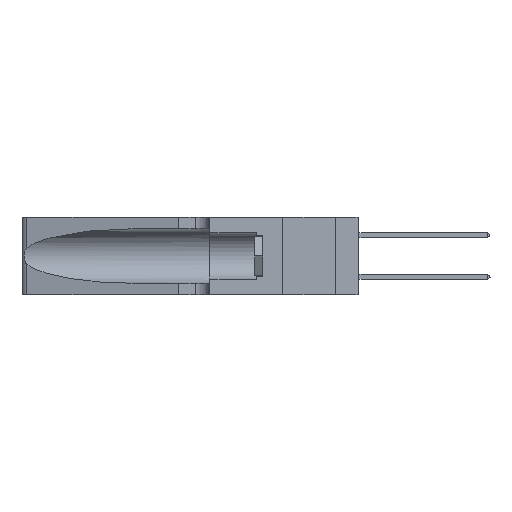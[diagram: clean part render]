
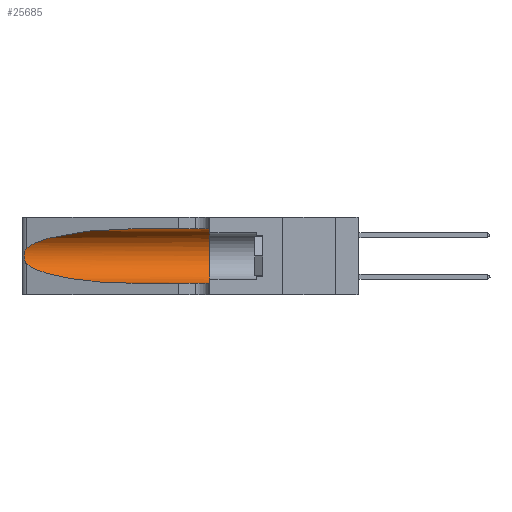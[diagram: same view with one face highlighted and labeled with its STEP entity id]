
A CAD part, left-side view. The second image highlights one B-rep face of the part: STEP entity #25685.
In plain terms, the highlighted cylindrical face has radius 3.308 mm (diameter 6.617 mm), a partial arc.
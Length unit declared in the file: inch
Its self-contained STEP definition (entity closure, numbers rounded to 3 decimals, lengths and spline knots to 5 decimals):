
#281 = CARTESIAN_POINT ( 'NONE',  ( 0.18966, 0.96281, 0.31525 ) ) ;
#1956 = CARTESIAN_POINT ( 'NONE',  ( 0.1305, 0.35, 0.185 ) ) ;
#2279 = VERTEX_POINT ( 'NONE', #17155 ) ;
#3001 = CARTESIAN_POINT ( 'NONE',  ( 0.25639, 1.23186, 0.15144 ) ) ;
#3052 = VERTEX_POINT ( 'NONE', #40512 ) ;
#3433 = VERTEX_POINT ( 'NONE', #13329 ) ;
#3722 = VERTEX_POINT ( 'NONE', #3764 ) ;
#3764 = CARTESIAN_POINT ( 'NONE',  ( 0.1305, 0.72297, 0.05475 ) ) ;
#4044 = ORIENTED_EDGE ( 'NONE', *, *, #33593, .T. ) ;
#4842 =( BOUNDED_CURVE ( )  B_SPLINE_CURVE ( 3, ( #26065, #281, #37174, #15163 ),
 .UNSPECIFIED., .F., .F. ) 
 B_SPLINE_CURVE_WITH_KNOTS ( ( 4, 4 ),
 ( 1.5708, 2.84003 ),
 .UNSPECIFIED. ) 
 CURVE ( )  GEOMETRIC_REPRESENTATION_ITEM ( )  RATIONAL_B_SPLINE_CURVE ( ( 1., 0.87, 0.87, 1. ) ) 
 REPRESENTATION_ITEM ( '' )  );
#5700 = DIRECTION ( 'NONE',  ( 0., 0., 1. ) ) ;
#6521 = CIRCLE ( 'NONE', #29920, 0.13025 ) ;
#6698 = AXIS2_PLACEMENT_3D ( 'NONE', #32342, #10132, #10285 ) ;
#6740 = CARTESIAN_POINT ( 'NONE',  ( 0.25487, 1.22718, 0.14631 ) ) ;
#8478 = VERTEX_POINT ( 'NONE', #41001 ) ;
#8802 = EDGE_CURVE ( 'NONE', #44204, #3433, #39065, .T. ) ;
#9090 = ORIENTED_EDGE ( 'NONE', *, *, #8802, .T. ) ;
#10132 = DIRECTION ( 'NONE',  ( 0., -1., 0. ) ) ;
#10261 = CARTESIAN_POINT ( 'NONE',  ( 0.25639, 1.23184, 0.21858 ) ) ;
#10285 = DIRECTION ( 'NONE',  ( 0., 0., -1. ) ) ;
#11110 = CARTESIAN_POINT ( 'NONE',  ( 0.18966, 0.96281, 0.05475 ) ) ;
#13057 = VECTOR ( 'NONE', #42154, 39.37008 ) ;
#13329 = CARTESIAN_POINT ( 'NONE',  ( 0.25487, 1.22718, 0.14631 ) ) ;
#13637 = VECTOR ( 'NONE', #43519, 39.37008 ) ;
#13995 = CARTESIAN_POINT ( 'NONE',  ( 0.25854, 1.2359, 0.20912 ) ) ;
#14206 = LINE ( 'NONE', #34748, #13057 ) ;
#15163 = CARTESIAN_POINT ( 'NONE',  ( 0.25487, 1.22718, 0.22369 ) ) ;
#17155 = CARTESIAN_POINT ( 'NONE',  ( 0.1305, 0.35, 0.05475 ) ) ;
#17729 = CARTESIAN_POINT ( 'NONE',  ( 0.26075, 1.23896, 0.19203 ) ) ;
#18454 =( BOUNDED_CURVE ( )  B_SPLINE_CURVE ( 3, ( #29433, #33156, #11110, #36834 ),
 .UNSPECIFIED., .F., .F. ) 
 B_SPLINE_CURVE_WITH_KNOTS ( ( 4, 4 ),
 ( 3.44316, 4.71239 ),
 .UNSPECIFIED. ) 
 CURVE ( )  GEOMETRIC_REPRESENTATION_ITEM ( )  RATIONAL_B_SPLINE_CURVE ( ( 1., 0.87, 0.87, 1. ) ) 
 REPRESENTATION_ITEM ( '' )  );
#19621 = EDGE_CURVE ( 'NONE', #3722, #2279, #23403, .T. ) ;
#21366 = CARTESIAN_POINT ( 'NONE',  ( 0.26017, 1.23833, 0.17102 ) ) ;
#21507 = EDGE_CURVE ( 'NONE', #8478, #2279, #6521, .T. ) ;
#21513 = CARTESIAN_POINT ( 'NONE',  ( 0.1305, 1.61858, 0.05475 ) ) ;
#21713 = CYLINDRICAL_SURFACE ( 'NONE', #6698, 0.13025 ) ;
#23403 = LINE ( 'NONE', #21513, #13637 ) ;
#25051 = CARTESIAN_POINT ( 'NONE',  ( 0.25789, 1.23486, 0.15765 ) ) ;
#25438 = EDGE_CURVE ( 'NONE', #3052, #8478, #14206, .T. ) ;
#25685 = ADVANCED_FACE ( 'NONE', ( #41280 ), #21713, .F. ) ;
#26065 = CARTESIAN_POINT ( 'NONE',  ( 0.1305, 0.72297, 0.31525 ) ) ;
#27713 = DIRECTION ( 'NONE',  ( 0., 1., 0. ) ) ;
#28762 = CARTESIAN_POINT ( 'NONE',  ( 0.25555, 1.22993, 0.14849 ) ) ;
#29433 = CARTESIAN_POINT ( 'NONE',  ( 0.25487, 1.22718, 0.14631 ) ) ;
#29920 = AXIS2_PLACEMENT_3D ( 'NONE', #1956, #27713, #5700 ) ;
#32315 = CARTESIAN_POINT ( 'NONE',  ( 0.25555, 1.22994, 0.2215 ) ) ;
#32342 = CARTESIAN_POINT ( 'NONE',  ( 0.1305, 1.61858, 0.185 ) ) ;
#33156 = CARTESIAN_POINT ( 'NONE',  ( 0.2373, 1.15595, 0.08982 ) ) ;
#33593 = EDGE_CURVE ( 'NONE', #3052, #44204, #4842, .T. ) ;
#34130 = ORIENTED_EDGE ( 'NONE', *, *, #19621, .T. ) ;
#34411 = ORIENTED_EDGE ( 'NONE', *, *, #42639, .T. ) ;
#34748 = CARTESIAN_POINT ( 'NONE',  ( 0.1305, 1.61858, 0.31525 ) ) ;
#35772 = EDGE_LOOP ( 'NONE', ( #4044, #9090, #34411, #34130, #37058, #37299 ) ) ;
#35986 = CARTESIAN_POINT ( 'NONE',  ( 0.25787, 1.23484, 0.2124 ) ) ;
#36834 = CARTESIAN_POINT ( 'NONE',  ( 0.1305, 0.72297, 0.05475 ) ) ;
#37058 = ORIENTED_EDGE ( 'NONE', *, *, #21507, .F. ) ;
#37174 = CARTESIAN_POINT ( 'NONE',  ( 0.2373, 1.15595, 0.28018 ) ) ;
#37299 = ORIENTED_EDGE ( 'NONE', *, *, #25438, .F. ) ;
#38891 = CARTESIAN_POINT ( 'NONE',  ( 0.25487, 1.22718, 0.22369 ) ) ;
#39065 = B_SPLINE_CURVE_WITH_KNOTS ( 'NONE', 3,
 ( #38891, #32315, #10261, #35986, #13995, #39690, #17729, #43375, #21366, #47042, #25051, #3001, #28762, #6740 ),
 .UNSPECIFIED., .F., .F.,
 ( 4, 2, 2, 2, 2, 2, 4 ),
 ( 0., 0.00027, 0.00053, 0.00107, 0.0016, 0.00187, 0.00214 ),
 .UNSPECIFIED. ) ;
#39690 = CARTESIAN_POINT ( 'NONE',  ( 0.26018, 1.23835, 0.19895 ) ) ;
#40512 = CARTESIAN_POINT ( 'NONE',  ( 0.1305, 0.72297, 0.31525 ) ) ;
#41001 = CARTESIAN_POINT ( 'NONE',  ( 0.1305, 0.35, 0.31525 ) ) ;
#41280 = FACE_OUTER_BOUND ( 'NONE', #35772, .T. ) ;
#42154 = DIRECTION ( 'NONE',  ( 0., -1., 0. ) ) ;
#42639 = EDGE_CURVE ( 'NONE', #3433, #3722, #18454, .T. ) ;
#43375 = CARTESIAN_POINT ( 'NONE',  ( 0.26075, 1.23896, 0.178 ) ) ;
#43519 = DIRECTION ( 'NONE',  ( 0., -1., 0. ) ) ;
#44204 = VERTEX_POINT ( 'NONE', #45356 ) ;
#45356 = CARTESIAN_POINT ( 'NONE',  ( 0.25487, 1.22718, 0.22369 ) ) ;
#47042 = CARTESIAN_POINT ( 'NONE',  ( 0.25856, 1.23593, 0.16098 ) ) ;
